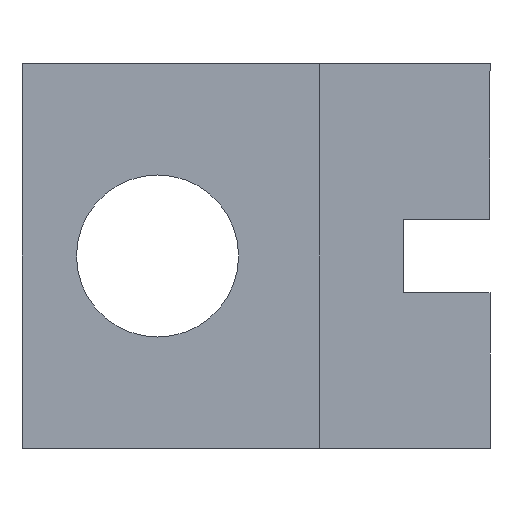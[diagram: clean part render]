
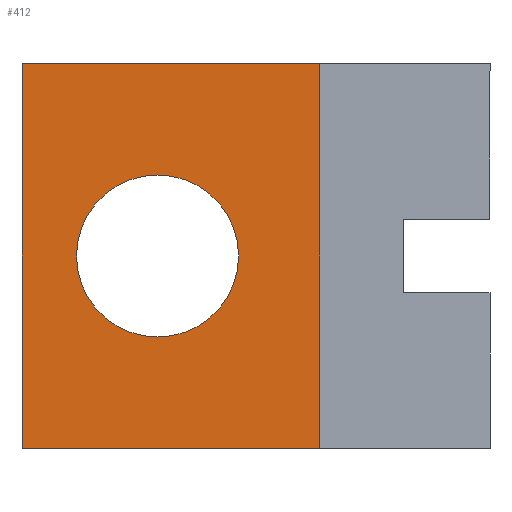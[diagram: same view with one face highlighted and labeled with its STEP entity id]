
A CAD part, front view. The second image highlights one B-rep face of the part: STEP entity #412.
In plain terms, the highlighted planar face has unit normal (0, -1, 0).
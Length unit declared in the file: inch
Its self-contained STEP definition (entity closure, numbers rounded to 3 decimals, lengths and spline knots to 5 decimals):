
#117 = CARTESIAN_POINT ( 'NONE',  ( 0.2865, 0., 0.37 ) ) ;
#138 = EDGE_CURVE ( 'NONE', #3309, #2651, #1291, .T. ) ;
#225 = CARTESIAN_POINT ( 'NONE',  ( 0.1305, 0., 0.107 ) ) ;
#336 = VECTOR ( 'NONE', #3812, 39.37008 ) ;
#353 = CARTESIAN_POINT ( 'NONE',  ( 0.2865, 0., 0. ) ) ;
#412 = ADVANCED_FACE ( 'NONE', ( #3038, #643 ), #2468, .F. ) ;
#417 = EDGE_CURVE ( 'NONE', #3739, #2288, #2450, .T. ) ;
#588 = ORIENTED_EDGE ( 'NONE', *, *, #3283, .F. ) ;
#597 = CARTESIAN_POINT ( 'NONE',  ( 0.1305, 0., 0.185 ) ) ;
#631 = DIRECTION ( 'NONE',  ( -1., 0., 0. ) ) ;
#643 = FACE_BOUND ( 'NONE', #2999, .T. ) ;
#670 = DIRECTION ( 'NONE',  ( 1., 0., 0. ) ) ;
#757 = VECTOR ( 'NONE', #670, 39.37008 ) ;
#1017 = ORIENTED_EDGE ( 'NONE', *, *, #417, .T. ) ;
#1073 = ORIENTED_EDGE ( 'NONE', *, *, #3099, .F. ) ;
#1249 = DIRECTION ( 'NONE',  ( -1., 0., 0. ) ) ;
#1291 = LINE ( 'NONE', #117, #3854 ) ;
#1354 = DIRECTION ( 'NONE',  ( 0., 0., -1. ) ) ;
#1372 = VERTEX_POINT ( 'NONE', #3569 ) ;
#1451 = AXIS2_PLACEMENT_3D ( 'NONE', #1809, #3101, #2725 ) ;
#1465 = EDGE_CURVE ( 'NONE', #2551, #1372, #2911, .T. ) ;
#1607 = CIRCLE ( 'NONE', #2497, 0.078 ) ;
#1809 = CARTESIAN_POINT ( 'NONE',  ( 0., 0., 0.37 ) ) ;
#1852 = CARTESIAN_POINT ( 'NONE',  ( 0., 0., 0.37 ) ) ;
#2052 = CARTESIAN_POINT ( 'NONE',  ( 0., 0., 0. ) ) ;
#2156 = LINE ( 'NONE', #2194, #757 ) ;
#2194 = CARTESIAN_POINT ( 'NONE',  ( 0., 0., 0. ) ) ;
#2288 = VERTEX_POINT ( 'NONE', #2052 ) ;
#2386 = DIRECTION ( 'NONE',  ( 0., -1., 0. ) ) ;
#2416 = EDGE_CURVE ( 'NONE', #2288, #2651, #2156, .T. ) ;
#2450 = LINE ( 'NONE', #1852, #3670 ) ;
#2468 = PLANE ( 'NONE',  #1451 ) ;
#2480 = DIRECTION ( 'NONE',  ( 0., -1., 0. ) ) ;
#2497 = AXIS2_PLACEMENT_3D ( 'NONE', #597, #2386, #1249 ) ;
#2510 = EDGE_LOOP ( 'NONE', ( #2838, #3501, #1073, #1017 ) ) ;
#2551 = VERTEX_POINT ( 'NONE', #225 ) ;
#2629 = CARTESIAN_POINT ( 'NONE',  ( 0., 0., 0.37 ) ) ;
#2651 = VERTEX_POINT ( 'NONE', #353 ) ;
#2685 = CARTESIAN_POINT ( 'NONE',  ( 0.2865, 0., 0.37 ) ) ;
#2722 = AXIS2_PLACEMENT_3D ( 'NONE', #3821, #2480, #631 ) ;
#2725 = DIRECTION ( 'NONE',  ( -1., 0., 0. ) ) ;
#2838 = ORIENTED_EDGE ( 'NONE', *, *, #2416, .T. ) ;
#2911 = CIRCLE ( 'NONE', #2722, 0.078 ) ;
#2999 = EDGE_LOOP ( 'NONE', ( #588, #3637 ) ) ;
#3038 = FACE_OUTER_BOUND ( 'NONE', #2510, .T. ) ;
#3099 = EDGE_CURVE ( 'NONE', #3739, #3309, #3255, .T. ) ;
#3101 = DIRECTION ( 'NONE',  ( 0., 1., 0. ) ) ;
#3255 = LINE ( 'NONE', #2629, #336 ) ;
#3283 = EDGE_CURVE ( 'NONE', #1372, #2551, #1607, .T. ) ;
#3309 = VERTEX_POINT ( 'NONE', #2685 ) ;
#3374 = DIRECTION ( 'NONE',  ( 0., 0., -1. ) ) ;
#3501 = ORIENTED_EDGE ( 'NONE', *, *, #138, .F. ) ;
#3569 = CARTESIAN_POINT ( 'NONE',  ( 0.1305, 0., 0.263 ) ) ;
#3582 = CARTESIAN_POINT ( 'NONE',  ( 0., 0., 0.37 ) ) ;
#3637 = ORIENTED_EDGE ( 'NONE', *, *, #1465, .F. ) ;
#3670 = VECTOR ( 'NONE', #3374, 39.37008 ) ;
#3739 = VERTEX_POINT ( 'NONE', #3582 ) ;
#3812 = DIRECTION ( 'NONE',  ( 1., 0., 0. ) ) ;
#3821 = CARTESIAN_POINT ( 'NONE',  ( 0.1305, 0., 0.185 ) ) ;
#3854 = VECTOR ( 'NONE', #1354, 39.37008 ) ;
